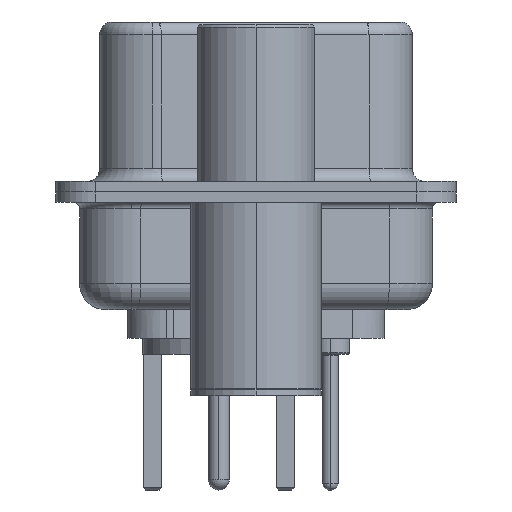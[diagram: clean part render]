
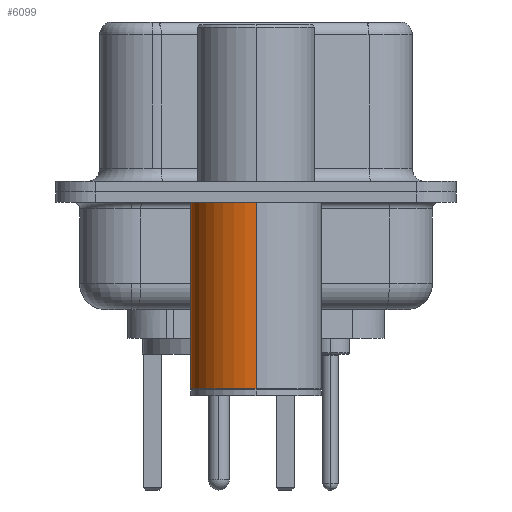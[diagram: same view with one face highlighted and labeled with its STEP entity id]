
A CAD part, left-side view. The second image highlights one B-rep face of the part: STEP entity #6099.
In plain terms, the highlighted cylindrical face has radius 2.5 mm (diameter 5 mm), a partial arc.
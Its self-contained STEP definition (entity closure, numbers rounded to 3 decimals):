
#264 = ORIENTED_EDGE ( 'NONE', *, *, #5841, .F. ) ;
#286 = VERTEX_POINT ( 'NONE', #19172 ) ;
#541 = DIRECTION ( 'NONE',  ( 0., 0., 1. ) ) ;
#1810 = LINE ( 'NONE', #16817, #11829 ) ;
#1864 = ORIENTED_EDGE ( 'NONE', *, *, #5777, .T. ) ;
#3083 = CARTESIAN_POINT ( 'NONE',  ( -2.5, 0., -7.525 ) ) ;
#3894 = ORIENTED_EDGE ( 'NONE', *, *, #5545, .T. ) ;
#4762 = DIRECTION ( 'NONE',  ( 1., 0., 0. ) ) ;
#4850 = DIRECTION ( 'NONE',  ( 0., 0., 1. ) ) ;
#4888 = CARTESIAN_POINT ( 'NONE',  ( 0., 0., -0.4 ) ) ;
#5545 = EDGE_CURVE ( 'NONE', #13152, #12531, #8473, .T. ) ;
#5777 = EDGE_CURVE ( 'NONE', #12531, #20192, #13373, .T. ) ;
#5841 = EDGE_CURVE ( 'NONE', #286, #20192, #16723, .T. ) ;
#5997 = EDGE_CURVE ( 'NONE', #13152, #286, #1810, .T. ) ;
#6099 = ADVANCED_FACE ( 'NONE', ( #24995 ), #9355, .T. ) ;
#6555 = CARTESIAN_POINT ( 'NONE',  ( -2.5, 0., 0.581 ) ) ;
#6644 = DIRECTION ( 'NONE',  ( 0., 0., 1. ) ) ;
#8212 = AXIS2_PLACEMENT_3D ( 'NONE', #4888, #4850, #4762 ) ;
#8473 = CIRCLE ( 'NONE', #13967, 2.5 ) ;
#9355 = CYLINDRICAL_SURFACE ( 'NONE', #19534, 2.5 ) ;
#9900 = CARTESIAN_POINT ( 'NONE',  ( -2.5, 0., -0.4 ) ) ;
#10956 = DIRECTION ( 'NONE',  ( 1., 0., 0. ) ) ;
#11005 = DIRECTION ( 'NONE',  ( 0., 0., 1. ) ) ;
#11044 = CARTESIAN_POINT ( 'NONE',  ( 0., 0., -7.525 ) ) ;
#11829 = VECTOR ( 'NONE', #541, 1000. ) ;
#12531 = VERTEX_POINT ( 'NONE', #3083 ) ;
#12667 = DIRECTION ( 'NONE',  ( 1., 0., 0. ) ) ;
#12857 = CARTESIAN_POINT ( 'NONE',  ( 2.5, 0., -7.525 ) ) ;
#13152 = VERTEX_POINT ( 'NONE', #12857 ) ;
#13373 = LINE ( 'NONE', #6555, #23163 ) ;
#13967 = AXIS2_PLACEMENT_3D ( 'NONE', #11044, #11005, #10956 ) ;
#14628 = CARTESIAN_POINT ( 'NONE',  ( 0., 0., 0.581 ) ) ;
#16723 = CIRCLE ( 'NONE', #8212, 2.5 ) ;
#16817 = CARTESIAN_POINT ( 'NONE',  ( 2.5, 0., 0.581 ) ) ;
#16911 = ORIENTED_EDGE ( 'NONE', *, *, #5997, .F. ) ;
#17183 = EDGE_LOOP ( 'NONE', ( #3894, #1864, #264, #16911 ) ) ;
#18494 = DIRECTION ( 'NONE',  ( 0., 0., 1. ) ) ;
#19172 = CARTESIAN_POINT ( 'NONE',  ( 2.5, 0., -0.4 ) ) ;
#19534 = AXIS2_PLACEMENT_3D ( 'NONE', #14628, #18494, #12667 ) ;
#20192 = VERTEX_POINT ( 'NONE', #9900 ) ;
#23163 = VECTOR ( 'NONE', #6644, 1000. ) ;
#24995 = FACE_OUTER_BOUND ( 'NONE', #17183, .T. ) ;
